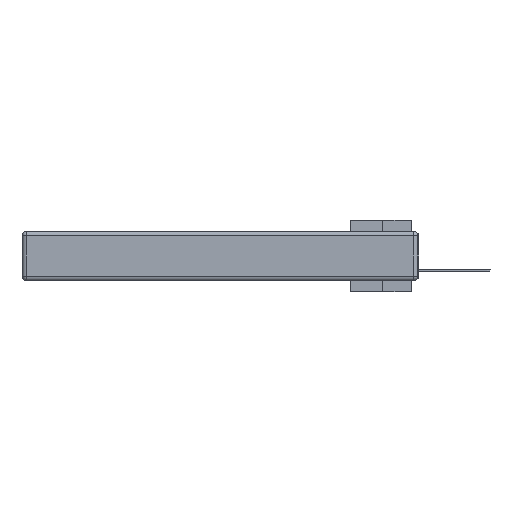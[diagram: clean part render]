
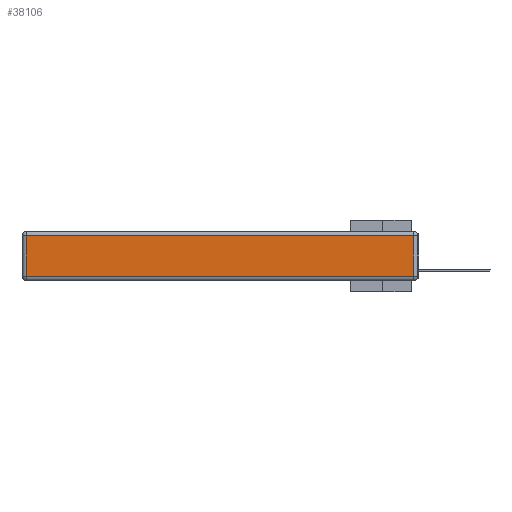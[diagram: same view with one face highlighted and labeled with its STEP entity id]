
A CAD part, left-side view. The second image highlights one B-rep face of the part: STEP entity #38106.
In plain terms, the highlighted planar face has unit normal (-1, 0, 0).
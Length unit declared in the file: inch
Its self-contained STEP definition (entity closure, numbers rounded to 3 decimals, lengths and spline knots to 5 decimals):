
#763 = VECTOR ( 'NONE', #30983, 39.37008 ) ;
#2894 = CARTESIAN_POINT ( 'NONE',  ( 0., 2.75, -0.03 ) ) ;
#4082 = ORIENTED_EDGE ( 'NONE', *, *, #35990, .T. ) ;
#4613 = CARTESIAN_POINT ( 'NONE',  ( 0., 2.72, -0.343 ) ) ;
#4762 = PLANE ( 'NONE',  #37616 ) ;
#4866 = FACE_OUTER_BOUND ( 'NONE', #30563, .T. ) ;
#5681 = EDGE_CURVE ( 'NONE', #16997, #35476, #33485, .T. ) ;
#6302 = CARTESIAN_POINT ( 'NONE',  ( 0., 2.72, -0.03 ) ) ;
#6334 = CARTESIAN_POINT ( 'NONE',  ( 0., 2.72, -0.313 ) ) ;
#9968 = CARTESIAN_POINT ( 'NONE',  ( 0., 0.03, -0.343 ) ) ;
#11688 = ORIENTED_EDGE ( 'NONE', *, *, #5681, .T. ) ;
#12035 = ORIENTED_EDGE ( 'NONE', *, *, #34206, .T. ) ;
#15391 = CARTESIAN_POINT ( 'NONE',  ( 0., 0.03, -0.313 ) ) ;
#16664 = CARTESIAN_POINT ( 'NONE',  ( 0., 0.03, -0.03 ) ) ;
#16900 = VERTEX_POINT ( 'NONE', #15391 ) ;
#16997 = VERTEX_POINT ( 'NONE', #6302 ) ;
#18141 = DIRECTION ( 'NONE',  ( 0., -1., 0. ) ) ;
#20392 = DIRECTION ( 'NONE',  ( 0., 1., 0. ) ) ;
#21047 = CARTESIAN_POINT ( 'NONE',  ( 0., 0., -0.313 ) ) ;
#22636 = CARTESIAN_POINT ( 'NONE',  ( 0., 0., -0.343 ) ) ;
#22741 = LINE ( 'NONE', #9968, #27435 ) ;
#25144 = ORIENTED_EDGE ( 'NONE', *, *, #29482, .T. ) ;
#25785 = DIRECTION ( 'NONE',  ( -1., 0., 0. ) ) ;
#25847 = VECTOR ( 'NONE', #20392, 39.37008 ) ;
#27435 = VECTOR ( 'NONE', #34406, 39.37008 ) ;
#28645 = DIRECTION ( 'NONE',  ( 0., 0., 1. ) ) ;
#29102 = LINE ( 'NONE', #2894, #25847 ) ;
#29482 = EDGE_CURVE ( 'NONE', #16900, #38747, #22741, .T. ) ;
#30563 = EDGE_LOOP ( 'NONE', ( #4082, #25144, #12035, #11688 ) ) ;
#30983 = DIRECTION ( 'NONE',  ( 0., 0., -1. ) ) ;
#32294 = LINE ( 'NONE', #21047, #35074 ) ;
#33485 = LINE ( 'NONE', #4613, #763 ) ;
#34206 = EDGE_CURVE ( 'NONE', #38747, #16997, #29102, .T. ) ;
#34406 = DIRECTION ( 'NONE',  ( 0., 0., 1. ) ) ;
#35074 = VECTOR ( 'NONE', #18141, 39.37008 ) ;
#35476 = VERTEX_POINT ( 'NONE', #6334 ) ;
#35990 = EDGE_CURVE ( 'NONE', #35476, #16900, #32294, .T. ) ;
#37616 = AXIS2_PLACEMENT_3D ( 'NONE', #22636, #25785, #28645 ) ;
#38106 = ADVANCED_FACE ( 'NONE', ( #4866 ), #4762, .T. ) ;
#38747 = VERTEX_POINT ( 'NONE', #16664 ) ;
